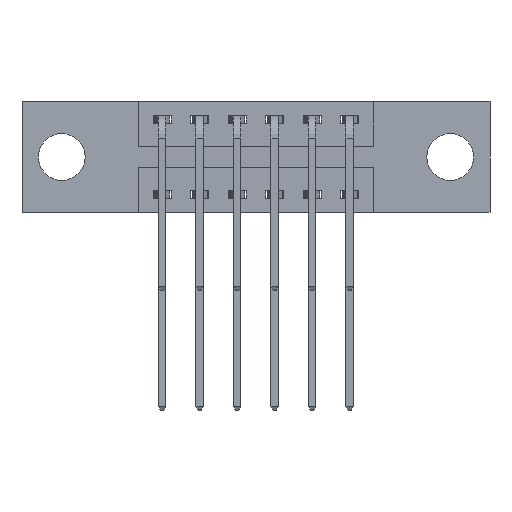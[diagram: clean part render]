
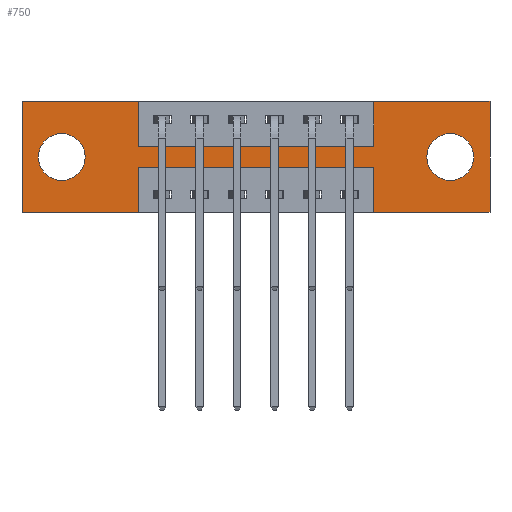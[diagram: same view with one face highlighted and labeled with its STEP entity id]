
A CAD part, front view. The second image highlights one B-rep face of the part: STEP entity #750.
In plain terms, the highlighted planar face has unit normal (0, -1, 0).
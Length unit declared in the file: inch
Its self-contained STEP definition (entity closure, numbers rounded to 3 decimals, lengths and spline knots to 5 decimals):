
#18 = VECTOR ( 'NONE', #1729, 39.37008 ) ;
#25 = EDGE_CURVE ( 'NONE', #2851, #6307, #4883, .T. ) ;
#78 = CARTESIAN_POINT ( 'NONE',  ( 0.1325, 0., -0.185 ) ) ;
#133 = CARTESIAN_POINT ( 'NONE',  ( 0., 0., -0.37 ) ) ;
#141 = CARTESIAN_POINT ( 'NONE',  ( 0.1325, 0., -0.263 ) ) ;
#153 = EDGE_CURVE ( 'NONE', #4748, #4223, #2740, .T. ) ;
#199 = CARTESIAN_POINT ( 'NONE',  ( 1.56, 0., 0. ) ) ;
#262 = DIRECTION ( 'NONE',  ( 0., 1., 0. ) ) ;
#264 = CARTESIAN_POINT ( 'NONE',  ( 1.1725, 0., -0.15 ) ) ;
#311 = CARTESIAN_POINT ( 'NONE',  ( 0., 0., 0. ) ) ;
#494 = CARTESIAN_POINT ( 'NONE',  ( 0., 0., -0.37 ) ) ;
#557 = LINE ( 'NONE', #8948, #1735 ) ;
#577 = DIRECTION ( 'NONE',  ( 0., 0., 1. ) ) ;
#641 = DIRECTION ( 'NONE',  ( 1., 0., 0. ) ) ;
#663 = DIRECTION ( 'NONE',  ( 0., 0., -1. ) ) ;
#675 = ORIENTED_EDGE ( 'NONE', *, *, #7684, .T. ) ;
#686 = CARTESIAN_POINT ( 'NONE',  ( 0.3875, 0., -0.15 ) ) ;
#750 = ADVANCED_FACE ( 'NONE', ( #3702, #1541, #9966 ), #5411, .T. ) ;
#792 = CARTESIAN_POINT ( 'NONE',  ( 0., 0., -0.37 ) ) ;
#883 = EDGE_CURVE ( 'NONE', #2229, #1250, #6047, .T. ) ;
#976 = CIRCLE ( 'NONE', #6107, 0.078 ) ;
#1005 = EDGE_LOOP ( 'NONE', ( #3459, #5412, #6104, #1282, #3528, #4065, #1552, #2078, #1324, #4104, #10082, #7526 ) ) ;
#1124 = EDGE_CURVE ( 'NONE', #6307, #2229, #7187, .T. ) ;
#1192 = EDGE_CURVE ( 'NONE', #3705, #3962, #1545, .T. ) ;
#1250 = VERTEX_POINT ( 'NONE', #264 ) ;
#1282 = ORIENTED_EDGE ( 'NONE', *, *, #153, .F. ) ;
#1324 = ORIENTED_EDGE ( 'NONE', *, *, #1124, .F. ) ;
#1541 = FACE_BOUND ( 'NONE', #8881, .T. ) ;
#1545 = LINE ( 'NONE', #792, #18 ) ;
#1552 = ORIENTED_EDGE ( 'NONE', *, *, #9316, .F. ) ;
#1559 = CARTESIAN_POINT ( 'NONE',  ( 0.3875, 0., -0.37 ) ) ;
#1634 = CARTESIAN_POINT ( 'NONE',  ( 0., 0., 0. ) ) ;
#1729 = DIRECTION ( 'NONE',  ( -1., 0., 0. ) ) ;
#1735 = VECTOR ( 'NONE', #663, 39.37008 ) ;
#1858 = CARTESIAN_POINT ( 'NONE',  ( 1.4275, 0., -0.185 ) ) ;
#1890 = DIRECTION ( 'NONE',  ( 0., 0., 1. ) ) ;
#2033 = VECTOR ( 'NONE', #3121, 39.37008 ) ;
#2078 = ORIENTED_EDGE ( 'NONE', *, *, #883, .F. ) ;
#2094 = VECTOR ( 'NONE', #8182, 39.37008 ) ;
#2120 = AXIS2_PLACEMENT_3D ( 'NONE', #78, #3287, #5815 ) ;
#2229 = VERTEX_POINT ( 'NONE', #8430 ) ;
#2351 = CARTESIAN_POINT ( 'NONE',  ( 0.3875, 0., -0.37 ) ) ;
#2371 = CARTESIAN_POINT ( 'NONE',  ( 0., 0., 0. ) ) ;
#2426 = CARTESIAN_POINT ( 'NONE',  ( 1.1725, 0., -0.22 ) ) ;
#2487 = CARTESIAN_POINT ( 'NONE',  ( 1.4275, 0., -0.263 ) ) ;
#2723 = CARTESIAN_POINT ( 'NONE',  ( 0., 0., -0.37 ) ) ;
#2740 = LINE ( 'NONE', #2723, #10496 ) ;
#2851 = VERTEX_POINT ( 'NONE', #3538 ) ;
#2996 = DIRECTION ( 'NONE',  ( 1., 0., 0. ) ) ;
#3121 = DIRECTION ( 'NONE',  ( 0., 0., 1. ) ) ;
#3153 = CARTESIAN_POINT ( 'NONE',  ( 0.1325, 0., -0.107 ) ) ;
#3287 = DIRECTION ( 'NONE',  ( 0., 1., 0. ) ) ;
#3359 = DIRECTION ( 'NONE',  ( 0., 0., -1. ) ) ;
#3380 = VERTEX_POINT ( 'NONE', #5581 ) ;
#3459 = ORIENTED_EDGE ( 'NONE', *, *, #8545, .F. ) ;
#3468 = VECTOR ( 'NONE', #9678, 39.37008 ) ;
#3480 = DIRECTION ( 'NONE',  ( 0., 0., -1. ) ) ;
#3509 = CARTESIAN_POINT ( 'NONE',  ( 1.4275, 0., -0.185 ) ) ;
#3528 = ORIENTED_EDGE ( 'NONE', *, *, #4811, .F. ) ;
#3538 = CARTESIAN_POINT ( 'NONE',  ( 0., 0., 0. ) ) ;
#3702 = FACE_BOUND ( 'NONE', #4240, .T. ) ;
#3705 = VERTEX_POINT ( 'NONE', #2351 ) ;
#3730 = LINE ( 'NONE', #6430, #3468 ) ;
#3827 = VERTEX_POINT ( 'NONE', #141 ) ;
#3962 = VERTEX_POINT ( 'NONE', #133 ) ;
#4065 = ORIENTED_EDGE ( 'NONE', *, *, #9268, .F. ) ;
#4079 = CARTESIAN_POINT ( 'NONE',  ( 1.1725, 0., -0.37 ) ) ;
#4104 = ORIENTED_EDGE ( 'NONE', *, *, #25, .F. ) ;
#4223 = VERTEX_POINT ( 'NONE', #4079 ) ;
#4240 = EDGE_LOOP ( 'NONE', ( #6826, #675 ) ) ;
#4354 = DIRECTION ( 'NONE',  ( 0., 0., -1. ) ) ;
#4442 = LINE ( 'NONE', #2371, #2033 ) ;
#4511 = CARTESIAN_POINT ( 'NONE',  ( 0.3875, 0., -0.22 ) ) ;
#4715 = EDGE_CURVE ( 'NONE', #4223, #9438, #5706, .T. ) ;
#4730 = VECTOR ( 'NONE', #3359, 39.37008 ) ;
#4748 = VERTEX_POINT ( 'NONE', #5424 ) ;
#4811 = EDGE_CURVE ( 'NONE', #7687, #4748, #557, .T. ) ;
#4883 = LINE ( 'NONE', #1634, #2094 ) ;
#4913 = VERTEX_POINT ( 'NONE', #2487 ) ;
#5005 = VECTOR ( 'NONE', #2996, 39.37008 ) ;
#5049 = VECTOR ( 'NONE', #1890, 39.37008 ) ;
#5144 = LINE ( 'NONE', #311, #8083 ) ;
#5362 = DIRECTION ( 'NONE',  ( -1., 0., 0. ) ) ;
#5411 = PLANE ( 'NONE',  #9038 ) ;
#5412 = ORIENTED_EDGE ( 'NONE', *, *, #5722, .F. ) ;
#5424 = CARTESIAN_POINT ( 'NONE',  ( 1.56, 0., -0.37 ) ) ;
#5581 = CARTESIAN_POINT ( 'NONE',  ( 1.1725, 0., 0. ) ) ;
#5641 = DIRECTION ( 'NONE',  ( 0., 0., -1. ) ) ;
#5706 = LINE ( 'NONE', #9176, #5049 ) ;
#5722 = EDGE_CURVE ( 'NONE', #9438, #8133, #8157, .T. ) ;
#5815 = DIRECTION ( 'NONE',  ( 0., 0., 1. ) ) ;
#5831 = VECTOR ( 'NONE', #5641, 39.37008 ) ;
#5995 = EDGE_CURVE ( 'NONE', #7026, #3827, #6650, .T. ) ;
#6047 = LINE ( 'NONE', #686, #5005 ) ;
#6104 = ORIENTED_EDGE ( 'NONE', *, *, #4715, .F. ) ;
#6107 = AXIS2_PLACEMENT_3D ( 'NONE', #3509, #262, #4354 ) ;
#6153 = DIRECTION ( 'NONE',  ( 0., -1., 0. ) ) ;
#6188 = AXIS2_PLACEMENT_3D ( 'NONE', #1858, #6780, #3480 ) ;
#6307 = VERTEX_POINT ( 'NONE', #8797 ) ;
#6342 = CARTESIAN_POINT ( 'NONE',  ( 1.4275, 0., -0.107 ) ) ;
#6372 = CARTESIAN_POINT ( 'NONE',  ( 0.1325, 0., -0.185 ) ) ;
#6399 = VECTOR ( 'NONE', #6997, 39.37008 ) ;
#6430 = CARTESIAN_POINT ( 'NONE',  ( 1.1725, 0., 0. ) ) ;
#6650 = CIRCLE ( 'NONE', #2120, 0.078 ) ;
#6741 = ORIENTED_EDGE ( 'NONE', *, *, #8365, .T. ) ;
#6780 = DIRECTION ( 'NONE',  ( 0., 1., 0. ) ) ;
#6826 = ORIENTED_EDGE ( 'NONE', *, *, #9502, .T. ) ;
#6997 = DIRECTION ( 'NONE',  ( -1., 0., 0. ) ) ;
#7026 = VERTEX_POINT ( 'NONE', #3153 ) ;
#7151 = AXIS2_PLACEMENT_3D ( 'NONE', #6372, #10325, #577 ) ;
#7187 = LINE ( 'NONE', #8321, #4730 ) ;
#7526 = ORIENTED_EDGE ( 'NONE', *, *, #1192, .F. ) ;
#7684 = EDGE_CURVE ( 'NONE', #4913, #8337, #976, .T. ) ;
#7687 = VERTEX_POINT ( 'NONE', #199 ) ;
#7753 = DIRECTION ( 'NONE',  ( 0., 0., -1. ) ) ;
#8083 = VECTOR ( 'NONE', #641, 39.37008 ) ;
#8133 = VERTEX_POINT ( 'NONE', #10334 ) ;
#8157 = LINE ( 'NONE', #4511, #6399 ) ;
#8182 = DIRECTION ( 'NONE',  ( 1., 0., 0. ) ) ;
#8321 = CARTESIAN_POINT ( 'NONE',  ( 0.3875, 0., 0. ) ) ;
#8337 = VERTEX_POINT ( 'NONE', #6342 ) ;
#8365 = EDGE_CURVE ( 'NONE', #3827, #7026, #9649, .T. ) ;
#8430 = CARTESIAN_POINT ( 'NONE',  ( 0.3875, 0., -0.15 ) ) ;
#8545 = EDGE_CURVE ( 'NONE', #8133, #3705, #9640, .T. ) ;
#8797 = CARTESIAN_POINT ( 'NONE',  ( 0.3875, 0., 0. ) ) ;
#8881 = EDGE_LOOP ( 'NONE', ( #9514, #6741 ) ) ;
#8948 = CARTESIAN_POINT ( 'NONE',  ( 1.56, 0., 0. ) ) ;
#9038 = AXIS2_PLACEMENT_3D ( 'NONE', #494, #6153, #7753 ) ;
#9176 = CARTESIAN_POINT ( 'NONE',  ( 1.1725, 0., -0.37 ) ) ;
#9225 = CIRCLE ( 'NONE', #6188, 0.078 ) ;
#9268 = EDGE_CURVE ( 'NONE', #3380, #7687, #5144, .T. ) ;
#9316 = EDGE_CURVE ( 'NONE', #1250, #3380, #3730, .T. ) ;
#9438 = VERTEX_POINT ( 'NONE', #2426 ) ;
#9502 = EDGE_CURVE ( 'NONE', #8337, #4913, #9225, .T. ) ;
#9514 = ORIENTED_EDGE ( 'NONE', *, *, #5995, .T. ) ;
#9640 = LINE ( 'NONE', #1559, #5831 ) ;
#9649 = CIRCLE ( 'NONE', #7151, 0.078 ) ;
#9678 = DIRECTION ( 'NONE',  ( 0., 0., 1. ) ) ;
#9966 = FACE_OUTER_BOUND ( 'NONE', #1005, .T. ) ;
#10082 = ORIENTED_EDGE ( 'NONE', *, *, #10211, .F. ) ;
#10211 = EDGE_CURVE ( 'NONE', #3962, #2851, #4442, .T. ) ;
#10325 = DIRECTION ( 'NONE',  ( 0., 1., 0. ) ) ;
#10334 = CARTESIAN_POINT ( 'NONE',  ( 0.3875, 0., -0.22 ) ) ;
#10496 = VECTOR ( 'NONE', #5362, 39.37008 ) ;
